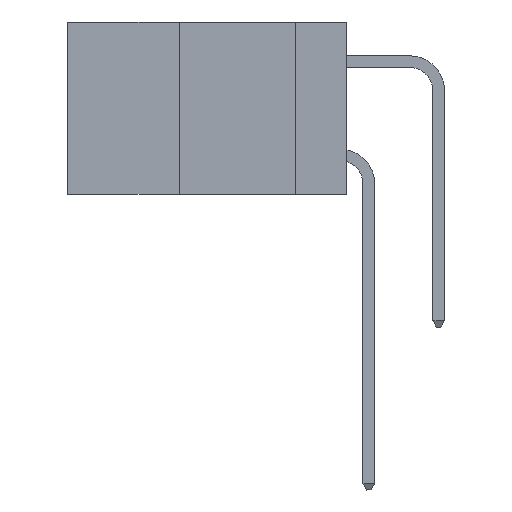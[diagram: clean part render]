
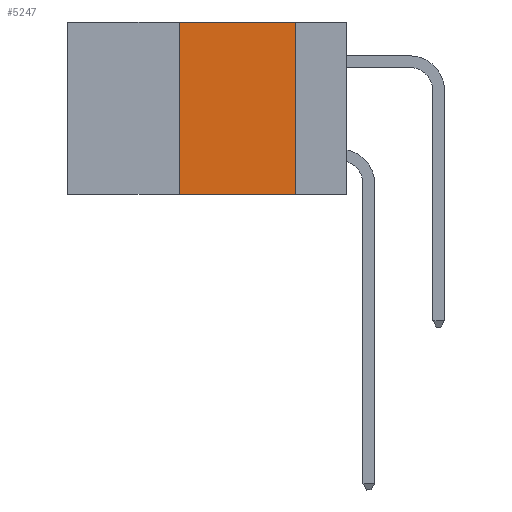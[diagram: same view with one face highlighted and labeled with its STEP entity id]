
A CAD part, left-side view. The second image highlights one B-rep face of the part: STEP entity #5247.
In plain terms, the highlighted planar face has unit normal (-1, 0, 0).
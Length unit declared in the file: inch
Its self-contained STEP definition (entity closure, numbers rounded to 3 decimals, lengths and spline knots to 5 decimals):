
#337 = VECTOR ( 'NONE', #22423, 39.37008 ) ;
#2232 = LINE ( 'NONE', #10297, #11539 ) ;
#3282 = EDGE_CURVE ( 'NONE', #25207, #5430, #14352, .T. ) ;
#5247 = ADVANCED_FACE ( 'NONE', ( #10769 ), #25994, .F. ) ;
#5430 = VERTEX_POINT ( 'NONE', #16861 ) ;
#6069 = VECTOR ( 'NONE', #19396, 39.37008 ) ;
#7387 = DIRECTION ( 'NONE',  ( 1., 0., 0. ) ) ;
#8092 = EDGE_LOOP ( 'NONE', ( #20855, #24546, #27420, #12239 ) ) ;
#9591 = EDGE_CURVE ( 'NONE', #13203, #25207, #19534, .T. ) ;
#10297 = CARTESIAN_POINT ( 'NONE',  ( 0., 0.36, 0. ) ) ;
#10769 = FACE_OUTER_BOUND ( 'NONE', #8092, .T. ) ;
#11539 = VECTOR ( 'NONE', #27646, 39.37008 ) ;
#12095 = VERTEX_POINT ( 'NONE', #17128 ) ;
#12239 = ORIENTED_EDGE ( 'NONE', *, *, #26918, .T. ) ;
#13203 = VERTEX_POINT ( 'NONE', #22428 ) ;
#13727 = CARTESIAN_POINT ( 'NONE',  ( 0., 0.6, -0.37 ) ) ;
#14352 = LINE ( 'NONE', #18778, #25351 ) ;
#14682 = CARTESIAN_POINT ( 'NONE',  ( 0., 0.6, 0. ) ) ;
#16861 = CARTESIAN_POINT ( 'NONE',  ( 0., 0.11, -0.37 ) ) ;
#17128 = CARTESIAN_POINT ( 'NONE',  ( 0., 0.36, -0.37 ) ) ;
#17716 = LINE ( 'NONE', #13727, #337 ) ;
#18778 = CARTESIAN_POINT ( 'NONE',  ( 0., 0.11, 0. ) ) ;
#19396 = DIRECTION ( 'NONE',  ( 0., -1., 0. ) ) ;
#19534 = LINE ( 'NONE', #14682, #6069 ) ;
#19762 = CARTESIAN_POINT ( 'NONE',  ( 0., 0.11, 0. ) ) ;
#20582 = CARTESIAN_POINT ( 'NONE',  ( 0., 0.6, 0. ) ) ;
#20855 = ORIENTED_EDGE ( 'NONE', *, *, #3282, .F. ) ;
#22423 = DIRECTION ( 'NONE',  ( 0., -1., 0. ) ) ;
#22428 = CARTESIAN_POINT ( 'NONE',  ( 0., 0.36, 0. ) ) ;
#22823 = EDGE_CURVE ( 'NONE', #12095, #13203, #2232, .T. ) ;
#24546 = ORIENTED_EDGE ( 'NONE', *, *, #9591, .F. ) ;
#25001 = DIRECTION ( 'NONE',  ( 0., 0., -1. ) ) ;
#25207 = VERTEX_POINT ( 'NONE', #19762 ) ;
#25351 = VECTOR ( 'NONE', #27444, 39.37008 ) ;
#25994 = PLANE ( 'NONE',  #27606 ) ;
#26918 = EDGE_CURVE ( 'NONE', #12095, #5430, #17716, .T. ) ;
#27420 = ORIENTED_EDGE ( 'NONE', *, *, #22823, .F. ) ;
#27444 = DIRECTION ( 'NONE',  ( 0., 0., -1. ) ) ;
#27606 = AXIS2_PLACEMENT_3D ( 'NONE', #20582, #7387, #25001 ) ;
#27646 = DIRECTION ( 'NONE',  ( 0., 0., 1. ) ) ;
